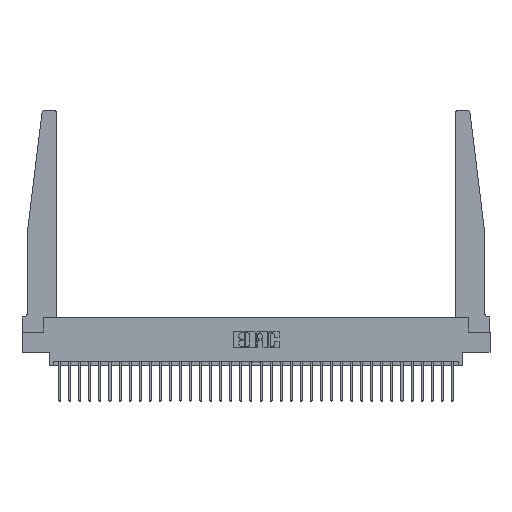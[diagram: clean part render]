
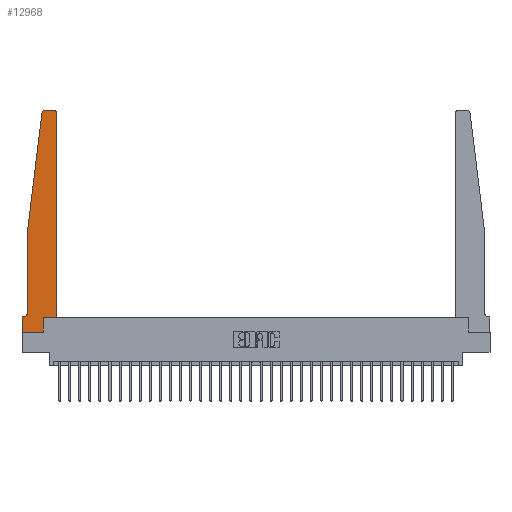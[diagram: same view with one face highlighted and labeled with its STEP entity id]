
A CAD part, top view. The second image highlights one B-rep face of the part: STEP entity #12968.
In plain terms, the highlighted planar face has unit normal (0, 0, 1).
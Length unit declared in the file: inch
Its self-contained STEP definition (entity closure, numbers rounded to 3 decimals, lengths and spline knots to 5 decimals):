
#82 = EDGE_CURVE ( 'NONE', #26381, #24589, #13826, .T. ) ;
#184 = CARTESIAN_POINT ( 'NONE',  ( 0.27653, 2.75, 0.37 ) ) ;
#472 = DIRECTION ( 'NONE',  ( 1., 0., 0. ) ) ;
#483 = CIRCLE ( 'NONE', #3036, 0.03 ) ;
#1934 = EDGE_CURVE ( 'NONE', #13831, #10377, #7610, .T. ) ;
#1945 = CARTESIAN_POINT ( 'NONE',  ( 0., 0.1875, 0.37 ) ) ;
#2458 = DIRECTION ( 'NONE',  ( 1., 0., 0. ) ) ;
#2532 = CARTESIAN_POINT ( 'NONE',  ( 0., 0.1875, 0.37 ) ) ;
#2642 = CARTESIAN_POINT ( 'NONE',  ( 0.065, 1.25, 0.37 ) ) ;
#3036 = AXIS2_PLACEMENT_3D ( 'NONE', #14525, #6804, #2458 ) ;
#3695 = DIRECTION ( 'NONE',  ( 0., -1., 0. ) ) ;
#3777 = ORIENTED_EDGE ( 'NONE', *, *, #12981, .T. ) ;
#3981 = ORIENTED_EDGE ( 'NONE', *, *, #5063, .T. ) ;
#4517 = CARTESIAN_POINT ( 'NONE',  ( 0.065, 1.25, 0.37 ) ) ;
#4834 = LINE ( 'NONE', #22182, #16423 ) ;
#4882 = CIRCLE ( 'NONE', #26953, 0.05 ) ;
#4914 = ORIENTED_EDGE ( 'NONE', *, *, #19258, .T. ) ;
#5063 = EDGE_CURVE ( 'NONE', #5597, #20796, #26527, .T. ) ;
#5135 = CARTESIAN_POINT ( 'NONE',  ( 0.2605, 0., 0.37 ) ) ;
#5597 = VERTEX_POINT ( 'NONE', #7687 ) ;
#5614 = CARTESIAN_POINT ( 'NONE',  ( 0.065, 0.1875, 0.37 ) ) ;
#6121 = VERTEX_POINT ( 'NONE', #14716 ) ;
#6244 = ORIENTED_EDGE ( 'NONE', *, *, #28792, .T. ) ;
#6740 = CARTESIAN_POINT ( 'NONE',  ( 0.2605, 0.18, 0.37 ) ) ;
#6750 = CARTESIAN_POINT ( 'NONE',  ( 0., 0., 0.37 ) ) ;
#6804 = DIRECTION ( 'NONE',  ( 0., 0., 1. ) ) ;
#7003 = CARTESIAN_POINT ( 'NONE',  ( 0.395, 2.75, 0.37 ) ) ;
#7610 = LINE ( 'NONE', #17423, #26182 ) ;
#7687 = CARTESIAN_POINT ( 'NONE',  ( 0.065, 1.25, 0.37 ) ) ;
#7877 = EDGE_CURVE ( 'NONE', #27241, #13831, #12192, .T. ) ;
#8800 = VECTOR ( 'NONE', #29709, 39.37008 ) ;
#9222 = CARTESIAN_POINT ( 'NONE',  ( 0., 0., 0.37 ) ) ;
#9360 = DIRECTION ( 'NONE',  ( 0., 0., 1. ) ) ;
#9878 = LINE ( 'NONE', #2642, #29615 ) ;
#10021 = CARTESIAN_POINT ( 'NONE',  ( 0.425, 0.18, 0.37 ) ) ;
#10343 = DIRECTION ( 'NONE',  ( -0.122, -0.992, 0. ) ) ;
#10377 = VERTEX_POINT ( 'NONE', #184 ) ;
#11624 = LINE ( 'NONE', #9222, #30528 ) ;
#11754 = DIRECTION ( 'NONE',  ( 0., 0., 1. ) ) ;
#12192 = CIRCLE ( 'NONE', #24002, 0.03 ) ;
#12232 = LINE ( 'NONE', #21861, #25869 ) ;
#12382 = EDGE_CURVE ( 'NONE', #10377, #6121, #483, .T. ) ;
#12968 = ADVANCED_FACE ( 'NONE', ( #14160 ), #26533, .T. ) ;
#12981 = EDGE_CURVE ( 'NONE', #31253, #27241, #4834, .T. ) ;
#13249 = DIRECTION ( 'NONE',  ( 0., 0., -1. ) ) ;
#13707 = DIRECTION ( 'NONE',  ( -1., 0., 0. ) ) ;
#13821 = LINE ( 'NONE', #6740, #26534 ) ;
#13826 = LINE ( 'NONE', #6750, #15352 ) ;
#13831 = VERTEX_POINT ( 'NONE', #7003 ) ;
#14160 = FACE_OUTER_BOUND ( 'NONE', #20516, .T. ) ;
#14330 = DIRECTION ( 'NONE',  ( 0., -1., 0. ) ) ;
#14525 = CARTESIAN_POINT ( 'NONE',  ( 0.27653, 2.72, 0.37 ) ) ;
#14716 = CARTESIAN_POINT ( 'NONE',  ( 0.24675, 2.72367, 0.37 ) ) ;
#15028 = VERTEX_POINT ( 'NONE', #25340 ) ;
#15352 = VECTOR ( 'NONE', #3695, 39.37008 ) ;
#15832 = CARTESIAN_POINT ( 'NONE',  ( 0.425, 2.72, 0.37 ) ) ;
#16423 = VECTOR ( 'NONE', #17380, 39.37008 ) ;
#16773 = ORIENTED_EDGE ( 'NONE', *, *, #7877, .T. ) ;
#16778 = EDGE_CURVE ( 'NONE', #24995, #26381, #27610, .T. ) ;
#17020 = CARTESIAN_POINT ( 'NONE',  ( 0.015, 0.1875, 0.37 ) ) ;
#17161 = ORIENTED_EDGE ( 'NONE', *, *, #19150, .T. ) ;
#17380 = DIRECTION ( 'NONE',  ( 0., 1., 0. ) ) ;
#17423 = CARTESIAN_POINT ( 'NONE',  ( 0.25, 2.75, 0.37 ) ) ;
#18901 = ORIENTED_EDGE ( 'NONE', *, *, #16778, .T. ) ;
#19150 = EDGE_CURVE ( 'NONE', #20796, #24995, #4882, .T. ) ;
#19155 = DIRECTION ( 'NONE',  ( 1., 0., 0. ) ) ;
#19258 = EDGE_CURVE ( 'NONE', #24589, #30305, #11624, .T. ) ;
#19510 = DIRECTION ( 'NONE',  ( -1., 0., 0. ) ) ;
#20010 = AXIS2_PLACEMENT_3D ( 'NONE', #1945, #11754, #21549 ) ;
#20516 = EDGE_LOOP ( 'NONE', ( #31681, #22242, #29663, #3981, #17161, #18901, #31150, #4914, #6244, #28720, #3777, #16773 ) ) ;
#20796 = VERTEX_POINT ( 'NONE', #29823 ) ;
#21549 = DIRECTION ( 'NONE',  ( 1., 0., 0. ) ) ;
#21861 = CARTESIAN_POINT ( 'NONE',  ( 0.425, 0.18, 0.37 ) ) ;
#22182 = CARTESIAN_POINT ( 'NONE',  ( 0.425, 0.18, 0.37 ) ) ;
#22242 = ORIENTED_EDGE ( 'NONE', *, *, #12382, .T. ) ;
#23762 = EDGE_CURVE ( 'NONE', #6121, #5597, #9878, .T. ) ;
#24002 = AXIS2_PLACEMENT_3D ( 'NONE', #31370, #9360, #19155 ) ;
#24395 = VECTOR ( 'NONE', #14330, 39.37008 ) ;
#24589 = VERTEX_POINT ( 'NONE', #31496 ) ;
#24995 = VERTEX_POINT ( 'NONE', #17020 ) ;
#25340 = CARTESIAN_POINT ( 'NONE',  ( 0.2605, 0.18, 0.37 ) ) ;
#25775 = CARTESIAN_POINT ( 'NONE',  ( 0.015, 0.2375, 0.37 ) ) ;
#25869 = VECTOR ( 'NONE', #472, 39.37008 ) ;
#25967 = EDGE_CURVE ( 'NONE', #15028, #31253, #12232, .T. ) ;
#26182 = VECTOR ( 'NONE', #19510, 39.37008 ) ;
#26381 = VERTEX_POINT ( 'NONE', #2532 ) ;
#26527 = LINE ( 'NONE', #4517, #24395 ) ;
#26533 = PLANE ( 'NONE',  #20010 ) ;
#26534 = VECTOR ( 'NONE', #30837, 39.37008 ) ;
#26953 = AXIS2_PLACEMENT_3D ( 'NONE', #25775, #13249, #13707 ) ;
#27241 = VERTEX_POINT ( 'NONE', #15832 ) ;
#27610 = LINE ( 'NONE', #5614, #8800 ) ;
#28720 = ORIENTED_EDGE ( 'NONE', *, *, #25967, .T. ) ;
#28792 = EDGE_CURVE ( 'NONE', #30305, #15028, #13821, .T. ) ;
#28813 = DIRECTION ( 'NONE',  ( 1., 0., 0. ) ) ;
#29615 = VECTOR ( 'NONE', #10343, 39.37008 ) ;
#29663 = ORIENTED_EDGE ( 'NONE', *, *, #23762, .T. ) ;
#29709 = DIRECTION ( 'NONE',  ( -1., 0., 0. ) ) ;
#29823 = CARTESIAN_POINT ( 'NONE',  ( 0.065, 0.2375, 0.37 ) ) ;
#30305 = VERTEX_POINT ( 'NONE', #5135 ) ;
#30528 = VECTOR ( 'NONE', #28813, 39.37008 ) ;
#30837 = DIRECTION ( 'NONE',  ( 0., 1., 0. ) ) ;
#31150 = ORIENTED_EDGE ( 'NONE', *, *, #82, .T. ) ;
#31253 = VERTEX_POINT ( 'NONE', #10021 ) ;
#31370 = CARTESIAN_POINT ( 'NONE',  ( 0.395, 2.72, 0.37 ) ) ;
#31496 = CARTESIAN_POINT ( 'NONE',  ( 0., 0., 0.37 ) ) ;
#31681 = ORIENTED_EDGE ( 'NONE', *, *, #1934, .T. ) ;
